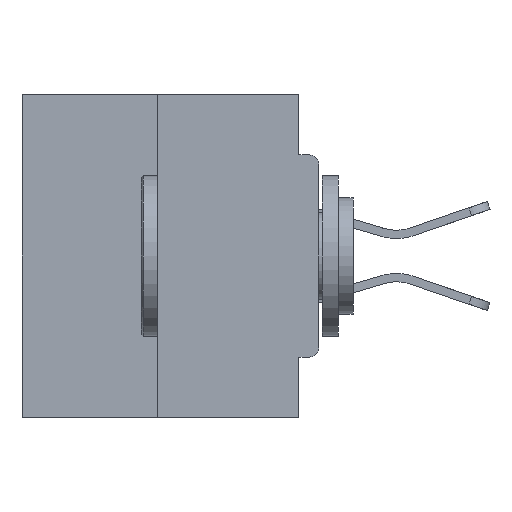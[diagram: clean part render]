
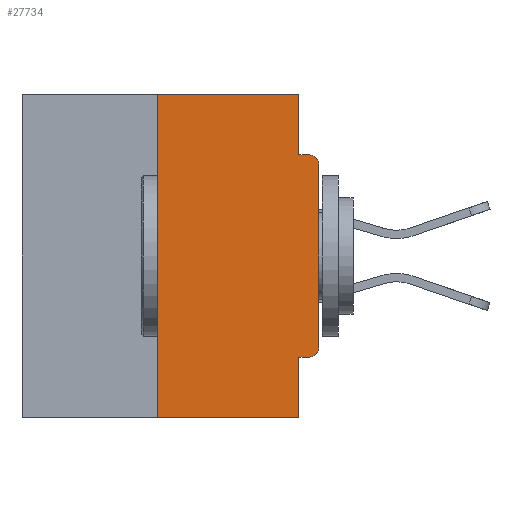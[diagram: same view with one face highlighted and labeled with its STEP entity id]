
A CAD part, left-side view. The second image highlights one B-rep face of the part: STEP entity #27734.
In plain terms, the highlighted planar face has unit normal (-1, 0, 0).
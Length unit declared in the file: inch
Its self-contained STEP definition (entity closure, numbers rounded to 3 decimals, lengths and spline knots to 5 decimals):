
#473 = DIRECTION ( 'NONE',  ( 0., 0., -1. ) ) ;
#985 = CARTESIAN_POINT ( 'NONE',  ( 0., 0.015, -0.4065 ) ) ;
#1123 = VERTEX_POINT ( 'NONE', #27976 ) ;
#2005 = AXIS2_PLACEMENT_3D ( 'NONE', #13540, #13198, #473 ) ;
#2612 = EDGE_CURVE ( 'NONE', #11509, #18573, #20115, .T. ) ;
#2687 = CARTESIAN_POINT ( 'NONE',  ( 0., 0., -0.1085 ) ) ;
#3001 = VECTOR ( 'NONE', #15421, 39.37008 ) ;
#3154 = EDGE_CURVE ( 'NONE', #29583, #26149, #5856, .T. ) ;
#3307 = DIRECTION ( 'NONE',  ( 0., 0., -1. ) ) ;
#3407 = ORIENTED_EDGE ( 'NONE', *, *, #25152, .F. ) ;
#3951 = LINE ( 'NONE', #13191, #4793 ) ;
#4431 = DIRECTION ( 'NONE',  ( 0., -1., 0. ) ) ;
#4793 = VECTOR ( 'NONE', #26025, 39.37008 ) ;
#4962 = VECTOR ( 'NONE', #24503, 39.37008 ) ;
#5198 = EDGE_CURVE ( 'NONE', #11509, #15302, #28861, .T. ) ;
#5481 = EDGE_CURVE ( 'NONE', #15302, #1123, #25188, .T. ) ;
#5749 = ORIENTED_EDGE ( 'NONE', *, *, #14648, .T. ) ;
#5856 = CIRCLE ( 'NONE', #13688, 0.015 ) ;
#7035 = CARTESIAN_POINT ( 'NONE',  ( 0., 0., -0.0935 ) ) ;
#7777 = LINE ( 'NONE', #29727, #4962 ) ;
#8182 = EDGE_CURVE ( 'NONE', #9326, #26149, #13245, .T. ) ;
#8240 = CARTESIAN_POINT ( 'NONE',  ( 0., 0.015, -0.3915 ) ) ;
#9326 = VERTEX_POINT ( 'NONE', #26508 ) ;
#10386 = EDGE_LOOP ( 'NONE', ( #3407, #32832, #5749, #22839, #23078, #16988, #33460, #22026, #14286, #26331 ) ) ;
#10567 = PLANE ( 'NONE',  #2005 ) ;
#10838 = VECTOR ( 'NONE', #15782, 39.37008 ) ;
#11509 = VERTEX_POINT ( 'NONE', #985 ) ;
#11783 = CARTESIAN_POINT ( 'NONE',  ( 0., 0.015, -0.0935 ) ) ;
#11853 = LINE ( 'NONE', #29213, #31002 ) ;
#13191 = CARTESIAN_POINT ( 'NONE',  ( 0., 0., 0. ) ) ;
#13198 = DIRECTION ( 'NONE',  ( 1., 0., 0. ) ) ;
#13245 = LINE ( 'NONE', #7035, #33200 ) ;
#13540 = CARTESIAN_POINT ( 'NONE',  ( 0., 0.46, 0. ) ) ;
#13688 = AXIS2_PLACEMENT_3D ( 'NONE', #23397, #18058, #33635 ) ;
#14286 = ORIENTED_EDGE ( 'NONE', *, *, #8182, .F. ) ;
#14558 = CARTESIAN_POINT ( 'NONE',  ( 0., 0.25, -0.5 ) ) ;
#14648 = EDGE_CURVE ( 'NONE', #28660, #1123, #7777, .T. ) ;
#15302 = VERTEX_POINT ( 'NONE', #22080 ) ;
#15388 = CARTESIAN_POINT ( 'NONE',  ( 0., 0.031, 0. ) ) ;
#15421 = DIRECTION ( 'NONE',  ( 0., -1., 0. ) ) ;
#15646 = VECTOR ( 'NONE', #28462, 39.37008 ) ;
#15746 = CARTESIAN_POINT ( 'NONE',  ( 0., 0.46, 0. ) ) ;
#15782 = DIRECTION ( 'NONE',  ( 0., 0., -1. ) ) ;
#15889 = CARTESIAN_POINT ( 'NONE',  ( 0., 0.031, -0.5 ) ) ;
#16073 = LINE ( 'NONE', #33294, #15646 ) ;
#16814 = FACE_OUTER_BOUND ( 'NONE', #10386, .T. ) ;
#16988 = ORIENTED_EDGE ( 'NONE', *, *, #2612, .T. ) ;
#18057 = LINE ( 'NONE', #15746, #3001 ) ;
#18058 = DIRECTION ( 'NONE',  ( -1., 0., 0. ) ) ;
#18294 = AXIS2_PLACEMENT_3D ( 'NONE', #8240, #18739, #26432 ) ;
#18573 = VERTEX_POINT ( 'NONE', #21857 ) ;
#18739 = DIRECTION ( 'NONE',  ( -1., 0., 0. ) ) ;
#20115 = CIRCLE ( 'NONE', #18294, 0.015 ) ;
#21857 = CARTESIAN_POINT ( 'NONE',  ( 0., 0., -0.3915 ) ) ;
#21962 = VECTOR ( 'NONE', #32521, 39.37008 ) ;
#22026 = ORIENTED_EDGE ( 'NONE', *, *, #3154, .T. ) ;
#22080 = CARTESIAN_POINT ( 'NONE',  ( 0., 0.031, -0.4065 ) ) ;
#22839 = ORIENTED_EDGE ( 'NONE', *, *, #5481, .F. ) ;
#23078 = ORIENTED_EDGE ( 'NONE', *, *, #5198, .F. ) ;
#23173 = VERTEX_POINT ( 'NONE', #31821 ) ;
#23397 = CARTESIAN_POINT ( 'NONE',  ( 0., 0.015, -0.1085 ) ) ;
#24503 = DIRECTION ( 'NONE',  ( 0., -1., 0. ) ) ;
#25152 = EDGE_CURVE ( 'NONE', #23173, #28161, #18057, .T. ) ;
#25188 = LINE ( 'NONE', #15889, #10838 ) ;
#25987 = EDGE_CURVE ( 'NONE', #28161, #9326, #11853, .T. ) ;
#26025 = DIRECTION ( 'NONE',  ( 0., 0., 1. ) ) ;
#26149 = VERTEX_POINT ( 'NONE', #11783 ) ;
#26331 = ORIENTED_EDGE ( 'NONE', *, *, #25987, .F. ) ;
#26432 = DIRECTION ( 'NONE',  ( 0., 0., -1. ) ) ;
#26508 = CARTESIAN_POINT ( 'NONE',  ( 0., 0.031, -0.0935 ) ) ;
#26952 = EDGE_CURVE ( 'NONE', #28660, #23173, #16073, .T. ) ;
#27734 = ADVANCED_FACE ( 'NONE', ( #16814 ), #10567, .F. ) ;
#27976 = CARTESIAN_POINT ( 'NONE',  ( 0., 0.031, -0.5 ) ) ;
#28161 = VERTEX_POINT ( 'NONE', #15388 ) ;
#28462 = DIRECTION ( 'NONE',  ( 0., 0., 1. ) ) ;
#28660 = VERTEX_POINT ( 'NONE', #14558 ) ;
#28861 = LINE ( 'NONE', #29885, #21962 ) ;
#29213 = CARTESIAN_POINT ( 'NONE',  ( 0., 0.031, 0. ) ) ;
#29583 = VERTEX_POINT ( 'NONE', #2687 ) ;
#29727 = CARTESIAN_POINT ( 'NONE',  ( 0., 0.46, -0.5 ) ) ;
#29885 = CARTESIAN_POINT ( 'NONE',  ( 0., 0., -0.4065 ) ) ;
#31002 = VECTOR ( 'NONE', #3307, 39.37008 ) ;
#31244 = EDGE_CURVE ( 'NONE', #18573, #29583, #3951, .T. ) ;
#31821 = CARTESIAN_POINT ( 'NONE',  ( 0., 0.25, 0. ) ) ;
#32521 = DIRECTION ( 'NONE',  ( 0., 1., 0. ) ) ;
#32832 = ORIENTED_EDGE ( 'NONE', *, *, #26952, .F. ) ;
#33200 = VECTOR ( 'NONE', #4431, 39.37008 ) ;
#33294 = CARTESIAN_POINT ( 'NONE',  ( 0., 0.25, 0. ) ) ;
#33460 = ORIENTED_EDGE ( 'NONE', *, *, #31244, .T. ) ;
#33635 = DIRECTION ( 'NONE',  ( 0., 0., -1. ) ) ;
